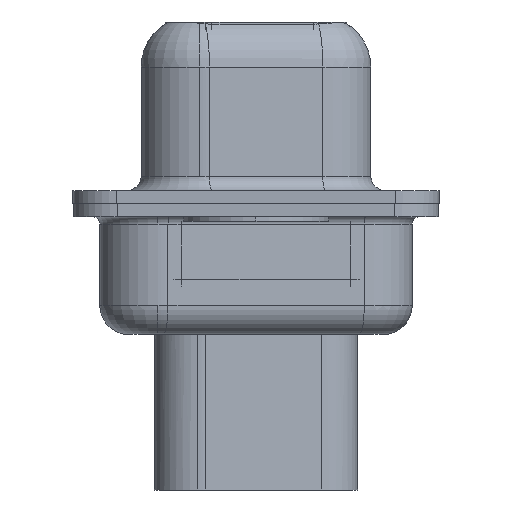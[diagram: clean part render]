
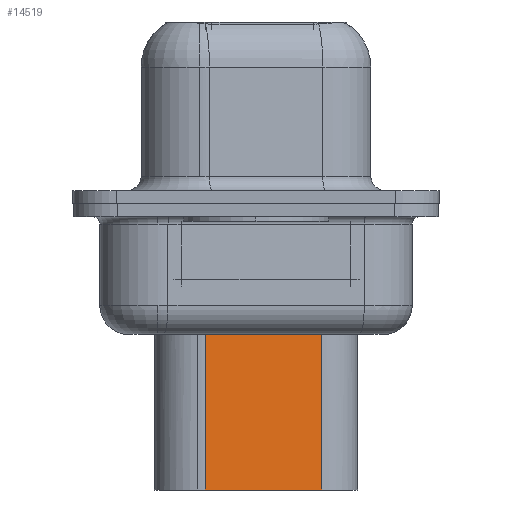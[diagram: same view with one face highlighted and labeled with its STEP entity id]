
A CAD part, left-side view. The second image highlights one B-rep face of the part: STEP entity #14519.
In plain terms, the highlighted planar face has unit normal (-0.985, -0.174, 0).
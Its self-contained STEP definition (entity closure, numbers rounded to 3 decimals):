
#35 = LINE ( 'NONE', #21320, #14089 ) ;
#326 = VECTOR ( 'NONE', #23654, 1000. ) ;
#1994 = CARTESIAN_POINT ( 'NONE',  ( 4.524, 1.74, -9.85 ) ) ;
#2611 = CARTESIAN_POINT ( 'NONE',  ( 4.524, 1.74, -3.1 ) ) ;
#4418 = LINE ( 'NONE', #1994, #9853 ) ;
#5129 = LINE ( 'NONE', #14405, #326 ) ;
#5857 = ORIENTED_EDGE ( 'NONE', *, *, #7917, .T. ) ;
#6552 = DIRECTION ( 'NONE',  ( -0.174, 0.985, 0. ) ) ;
#7508 = ORIENTED_EDGE ( 'NONE', *, *, #22861, .T. ) ;
#7917 = EDGE_CURVE ( 'NONE', #26474, #9486, #17870, .T. ) ;
#8127 = AXIS2_PLACEMENT_3D ( 'NONE', #2611, #14306, #11881 ) ;
#9486 = VERTEX_POINT ( 'NONE', #24952 ) ;
#9495 = VERTEX_POINT ( 'NONE', #27231 ) ;
#9853 = VECTOR ( 'NONE', #6552, 1000. ) ;
#10809 = CARTESIAN_POINT ( 'NONE',  ( 5.229, -2.26, -9.85 ) ) ;
#11881 = DIRECTION ( 'NONE',  ( 0.174, -0.985, 0. ) ) ;
#12856 = DIRECTION ( 'NONE',  ( -0.174, 0.985, 0. ) ) ;
#14089 = VECTOR ( 'NONE', #26010, 1000. ) ;
#14306 = DIRECTION ( 'NONE',  ( -0.985, -0.174, 0. ) ) ;
#14405 = CARTESIAN_POINT ( 'NONE',  ( 4.524, 1.74, -3.1 ) ) ;
#14443 = ORIENTED_EDGE ( 'NONE', *, *, #28300, .F. ) ;
#14519 = ADVANCED_FACE ( 'NONE', ( #16143 ), #18878, .T. ) ;
#15722 = VECTOR ( 'NONE', #12856, 1000. ) ;
#16143 = FACE_OUTER_BOUND ( 'NONE', #25593, .T. ) ;
#17429 = CARTESIAN_POINT ( 'NONE',  ( 4.353, 2.709, -3.975 ) ) ;
#17870 = LINE ( 'NONE', #17429, #15722 ) ;
#17963 = CARTESIAN_POINT ( 'NONE',  ( 5.229, -2.26, -3.975 ) ) ;
#18878 = PLANE ( 'NONE',  #8127 ) ;
#21196 = ORIENTED_EDGE ( 'NONE', *, *, #24863, .F. ) ;
#21320 = CARTESIAN_POINT ( 'NONE',  ( 5.229, -2.26, -3.1 ) ) ;
#22861 = EDGE_CURVE ( 'NONE', #9486, #9495, #5129, .T. ) ;
#23654 = DIRECTION ( 'NONE',  ( 0., 0., -1. ) ) ;
#23987 = VERTEX_POINT ( 'NONE', #10809 ) ;
#24863 = EDGE_CURVE ( 'NONE', #26474, #23987, #35, .T. ) ;
#24952 = CARTESIAN_POINT ( 'NONE',  ( 4.524, 1.74, -3.975 ) ) ;
#25593 = EDGE_LOOP ( 'NONE', ( #21196, #5857, #7508, #14443 ) ) ;
#26010 = DIRECTION ( 'NONE',  ( 0., 0., -1. ) ) ;
#26474 = VERTEX_POINT ( 'NONE', #17963 ) ;
#27231 = CARTESIAN_POINT ( 'NONE',  ( 4.524, 1.74, -9.85 ) ) ;
#28300 = EDGE_CURVE ( 'NONE', #23987, #9495, #4418, .T. ) ;
